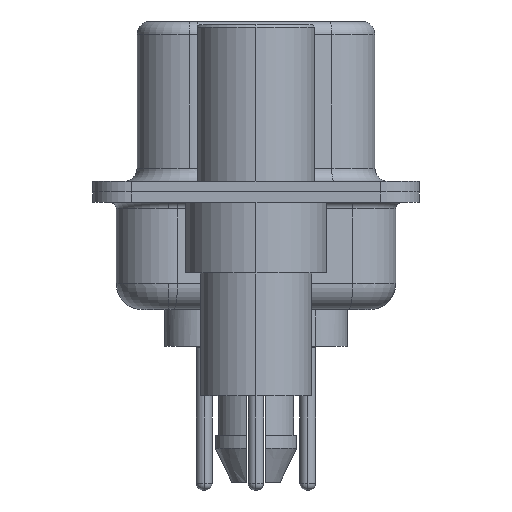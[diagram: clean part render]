
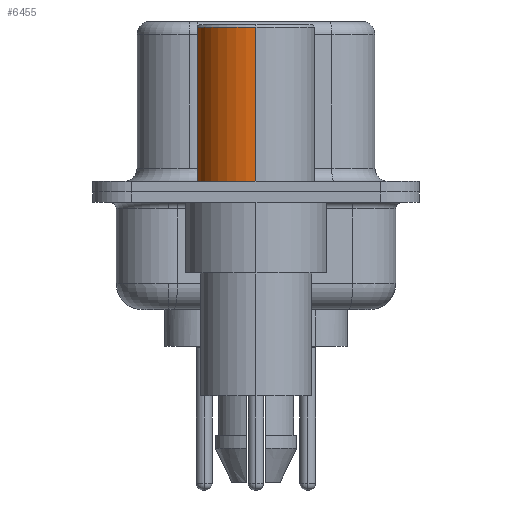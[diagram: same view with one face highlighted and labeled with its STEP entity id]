
A CAD part, left-side view. The second image highlights one B-rep face of the part: STEP entity #6455.
In plain terms, the highlighted cylindrical face has radius 2.25 mm (diameter 4.5 mm), a partial arc.
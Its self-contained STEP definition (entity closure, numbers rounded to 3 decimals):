
#112 = VECTOR ( 'NONE', #6085, 1000. ) ;
#182 = AXIS2_PLACEMENT_3D ( 'NONE', #16714, #6713, #18306 ) ;
#642 = CARTESIAN_POINT ( 'NONE',  ( 0., 0., 6.3 ) ) ;
#1301 = EDGE_LOOP ( 'NONE', ( #14808, #20625, #14344, #16430 ) ) ;
#1648 = DIRECTION ( 'NONE',  ( 0., 0., 1. ) ) ;
#1727 = VERTEX_POINT ( 'NONE', #12828 ) ;
#2363 = DIRECTION ( 'NONE',  ( 1., 0., 0. ) ) ;
#3886 = EDGE_CURVE ( 'NONE', #7617, #14782, #5724, .T. ) ;
#4328 = CARTESIAN_POINT ( 'NONE',  ( 0., 0., 0.581 ) ) ;
#4504 = VECTOR ( 'NONE', #19862, 1000. ) ;
#5724 = LINE ( 'NONE', #5882, #112 ) ;
#5882 = CARTESIAN_POINT ( 'NONE',  ( -2.25, 0., 0.581 ) ) ;
#5977 = CYLINDRICAL_SURFACE ( 'NONE', #20770, 2.25 ) ;
#6085 = DIRECTION ( 'NONE',  ( 0., 0., 1. ) ) ;
#6353 = CARTESIAN_POINT ( 'NONE',  ( 2.25, 0., 6.3 ) ) ;
#6455 = ADVANCED_FACE ( 'NONE', ( #10084 ), #5977, .T. ) ;
#6713 = DIRECTION ( 'NONE',  ( 0., 0., 1. ) ) ;
#7617 = VERTEX_POINT ( 'NONE', #17576 ) ;
#10084 = FACE_OUTER_BOUND ( 'NONE', #1301, .T. ) ;
#12064 = CIRCLE ( 'NONE', #19839, 2.25 ) ;
#12473 = DIRECTION ( 'NONE',  ( 0., 0., 1. ) ) ;
#12828 = CARTESIAN_POINT ( 'NONE',  ( 2.25, 0., 0.4 ) ) ;
#13563 = CIRCLE ( 'NONE', #182, 2.25 ) ;
#14344 = ORIENTED_EDGE ( 'NONE', *, *, #15605, .F. ) ;
#14782 = VERTEX_POINT ( 'NONE', #18388 ) ;
#14808 = ORIENTED_EDGE ( 'NONE', *, *, #17144, .T. ) ;
#15225 = VERTEX_POINT ( 'NONE', #6353 ) ;
#15605 = EDGE_CURVE ( 'NONE', #15225, #14782, #12064, .T. ) ;
#16430 = ORIENTED_EDGE ( 'NONE', *, *, #19931, .F. ) ;
#16714 = CARTESIAN_POINT ( 'NONE',  ( 0., 0., 0.4 ) ) ;
#17144 = EDGE_CURVE ( 'NONE', #1727, #7617, #13563, .T. ) ;
#17576 = CARTESIAN_POINT ( 'NONE',  ( -2.25, 0., 0.4 ) ) ;
#17646 = DIRECTION ( 'NONE',  ( 1., 0., 0. ) ) ;
#18262 = CARTESIAN_POINT ( 'NONE',  ( 2.25, 0., 0.581 ) ) ;
#18306 = DIRECTION ( 'NONE',  ( 1., 0., 0. ) ) ;
#18388 = CARTESIAN_POINT ( 'NONE',  ( -2.25, 0., 6.3 ) ) ;
#19839 = AXIS2_PLACEMENT_3D ( 'NONE', #642, #12473, #2363 ) ;
#19862 = DIRECTION ( 'NONE',  ( 0., 0., 1. ) ) ;
#19931 = EDGE_CURVE ( 'NONE', #1727, #15225, #21492, .T. ) ;
#20625 = ORIENTED_EDGE ( 'NONE', *, *, #3886, .T. ) ;
#20770 = AXIS2_PLACEMENT_3D ( 'NONE', #4328, #1648, #17646 ) ;
#21492 = LINE ( 'NONE', #18262, #4504 ) ;
